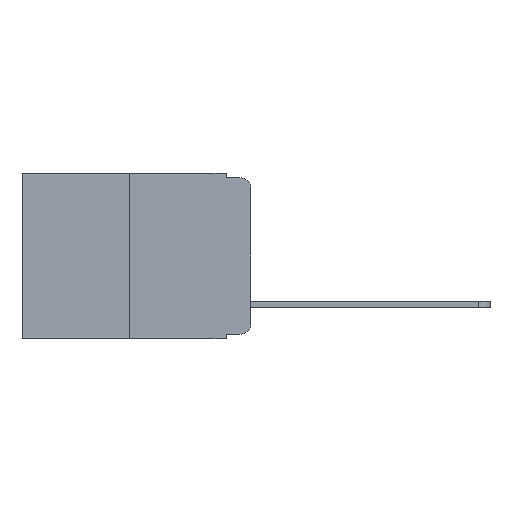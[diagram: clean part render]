
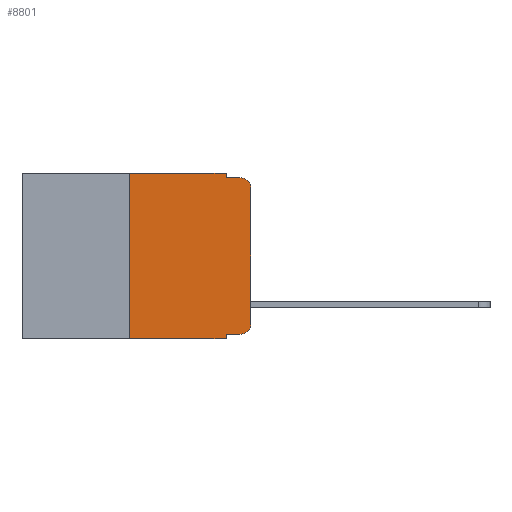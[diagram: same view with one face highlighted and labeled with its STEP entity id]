
A CAD part, left-side view. The second image highlights one B-rep face of the part: STEP entity #8801.
In plain terms, the highlighted planar face has unit normal (-1, 0, 0).
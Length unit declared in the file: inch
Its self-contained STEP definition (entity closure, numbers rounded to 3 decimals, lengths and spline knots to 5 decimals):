
#96 = VERTEX_POINT ( 'NONE', #7176 ) ;
#992 = DIRECTION ( 'NONE',  ( 0., 0., -1. ) ) ;
#1319 = DIRECTION ( 'NONE',  ( 0., -1., 0. ) ) ;
#1558 = CARTESIAN_POINT ( 'NONE',  ( 0., 0.051, 0. ) ) ;
#1704 = VECTOR ( 'NONE', #992, 39.37008 ) ;
#1750 = CARTESIAN_POINT ( 'NONE',  ( 0., 0.051, -0.343 ) ) ;
#1801 = VECTOR ( 'NONE', #6976, 39.37008 ) ;
#1995 = VERTEX_POINT ( 'NONE', #7747 ) ;
#1996 = VERTEX_POINT ( 'NONE', #17955 ) ;
#2219 = DIRECTION ( 'NONE',  ( 0., 0., -1. ) ) ;
#2362 = CARTESIAN_POINT ( 'NONE',  ( 0., 0.051, -0.01 ) ) ;
#2568 = ORIENTED_EDGE ( 'NONE', *, *, #17423, .T. ) ;
#2711 = VERTEX_POINT ( 'NONE', #15989 ) ;
#2760 = ORIENTED_EDGE ( 'NONE', *, *, #4101, .T. ) ;
#3169 = VECTOR ( 'NONE', #3296, 39.37008 ) ;
#3296 = DIRECTION ( 'NONE',  ( 0., 0., 1. ) ) ;
#3341 = CARTESIAN_POINT ( 'NONE',  ( 0., 0.473, -0.343 ) ) ;
#3750 = AXIS2_PLACEMENT_3D ( 'NONE', #8411, #7638, #8031 ) ;
#4101 = EDGE_CURVE ( 'NONE', #12578, #96, #6344, .T. ) ;
#4125 = VECTOR ( 'NONE', #1319, 39.37008 ) ;
#4713 = AXIS2_PLACEMENT_3D ( 'NONE', #14278, #5470, #15530 ) ;
#5449 = LINE ( 'NONE', #14874, #9490 ) ;
#5470 = DIRECTION ( 'NONE',  ( -1., 0., 0. ) ) ;
#5997 = LINE ( 'NONE', #1558, #1704 ) ;
#6018 = DIRECTION ( 'NONE',  ( 0., 0., 1. ) ) ;
#6344 = CIRCLE ( 'NONE', #17458, 0.02 ) ;
#6750 = EDGE_CURVE ( 'NONE', #14552, #10929, #12159, .T. ) ;
#6965 = CARTESIAN_POINT ( 'NONE',  ( 0., 0.051, -0.333 ) ) ;
#6976 = DIRECTION ( 'NONE',  ( 0., 0., -1. ) ) ;
#7154 = CARTESIAN_POINT ( 'NONE',  ( 0., 0., -0.03 ) ) ;
#7176 = CARTESIAN_POINT ( 'NONE',  ( 0., 0.02, -0.01 ) ) ;
#7191 = CARTESIAN_POINT ( 'NONE',  ( 0., 0.051, 0. ) ) ;
#7440 = DIRECTION ( 'NONE',  ( -1., 0., 0. ) ) ;
#7570 = ORIENTED_EDGE ( 'NONE', *, *, #8406, .F. ) ;
#7609 = PLANE ( 'NONE',  #3750 ) ;
#7638 = DIRECTION ( 'NONE',  ( 1., 0., 0. ) ) ;
#7747 = CARTESIAN_POINT ( 'NONE',  ( 0., 0.25, -0.343 ) ) ;
#8031 = DIRECTION ( 'NONE',  ( 0., 0., -1. ) ) ;
#8220 = CARTESIAN_POINT ( 'NONE',  ( 0., 0.051, -0.01 ) ) ;
#8406 = EDGE_CURVE ( 'NONE', #14552, #17861, #9668, .T. ) ;
#8411 = CARTESIAN_POINT ( 'NONE',  ( 0., 0.473, 0. ) ) ;
#8785 = VERTEX_POINT ( 'NONE', #8220 ) ;
#8801 = ADVANCED_FACE ( 'NONE', ( #10555 ), #7609, .F. ) ;
#8996 = ORIENTED_EDGE ( 'NONE', *, *, #6750, .T. ) ;
#9210 = ORIENTED_EDGE ( 'NONE', *, *, #17859, .T. ) ;
#9490 = VECTOR ( 'NONE', #6018, 39.37008 ) ;
#9549 = EDGE_LOOP ( 'NONE', ( #13047, #2760, #12831, #10816, #9920, #10350, #9210, #7570, #8996, #2568 ) ) ;
#9668 = LINE ( 'NONE', #7191, #1801 ) ;
#9766 = CARTESIAN_POINT ( 'NONE',  ( 0., 0.473, 0. ) ) ;
#9920 = ORIENTED_EDGE ( 'NONE', *, *, #13372, .F. ) ;
#10145 = CARTESIAN_POINT ( 'NONE',  ( 0., 0.02, -0.03 ) ) ;
#10176 = DIRECTION ( 'NONE',  ( 0., -1., 0. ) ) ;
#10350 = ORIENTED_EDGE ( 'NONE', *, *, #13884, .F. ) ;
#10555 = FACE_OUTER_BOUND ( 'NONE', #9549, .T. ) ;
#10651 = EDGE_CURVE ( 'NONE', #17076, #8785, #5997, .T. ) ;
#10816 = ORIENTED_EDGE ( 'NONE', *, *, #10651, .F. ) ;
#10929 = VERTEX_POINT ( 'NONE', #13291 ) ;
#11925 = VECTOR ( 'NONE', #15172, 39.37008 ) ;
#12056 = CARTESIAN_POINT ( 'NONE',  ( 0., 0.051, 0. ) ) ;
#12159 = LINE ( 'NONE', #12990, #4125 ) ;
#12205 = EDGE_CURVE ( 'NONE', #2711, #12578, #5449, .T. ) ;
#12578 = VERTEX_POINT ( 'NONE', #7154 ) ;
#12585 = EDGE_CURVE ( 'NONE', #8785, #96, #12587, .T. ) ;
#12587 = LINE ( 'NONE', #2362, #15693 ) ;
#12609 = CIRCLE ( 'NONE', #4713, 0.02 ) ;
#12831 = ORIENTED_EDGE ( 'NONE', *, *, #12585, .F. ) ;
#12990 = CARTESIAN_POINT ( 'NONE',  ( 0., 0.051, -0.333 ) ) ;
#13047 = ORIENTED_EDGE ( 'NONE', *, *, #12205, .T. ) ;
#13291 = CARTESIAN_POINT ( 'NONE',  ( 0., 0.02, -0.333 ) ) ;
#13372 = EDGE_CURVE ( 'NONE', #1996, #17076, #14474, .T. ) ;
#13884 = EDGE_CURVE ( 'NONE', #1995, #1996, #15027, .T. ) ;
#14278 = CARTESIAN_POINT ( 'NONE',  ( 0., 0.02, -0.313 ) ) ;
#14474 = LINE ( 'NONE', #9766, #17482 ) ;
#14552 = VERTEX_POINT ( 'NONE', #6965 ) ;
#14874 = CARTESIAN_POINT ( 'NONE',  ( 0., 0., 0. ) ) ;
#15027 = LINE ( 'NONE', #16389, #3169 ) ;
#15172 = DIRECTION ( 'NONE',  ( 0., -1., 0. ) ) ;
#15530 = DIRECTION ( 'NONE',  ( 0., 0., -1. ) ) ;
#15693 = VECTOR ( 'NONE', #10176, 39.37008 ) ;
#15989 = CARTESIAN_POINT ( 'NONE',  ( 0., 0., -0.313 ) ) ;
#16389 = CARTESIAN_POINT ( 'NONE',  ( 0., 0.25, 0. ) ) ;
#17076 = VERTEX_POINT ( 'NONE', #12056 ) ;
#17423 = EDGE_CURVE ( 'NONE', #10929, #2711, #12609, .T. ) ;
#17458 = AXIS2_PLACEMENT_3D ( 'NONE', #10145, #7440, #2219 ) ;
#17482 = VECTOR ( 'NONE', #17872, 39.37008 ) ;
#17859 = EDGE_CURVE ( 'NONE', #1995, #17861, #18526, .T. ) ;
#17861 = VERTEX_POINT ( 'NONE', #1750 ) ;
#17872 = DIRECTION ( 'NONE',  ( 0., -1., 0. ) ) ;
#17955 = CARTESIAN_POINT ( 'NONE',  ( 0., 0.25, 0. ) ) ;
#18526 = LINE ( 'NONE', #3341, #11925 ) ;
